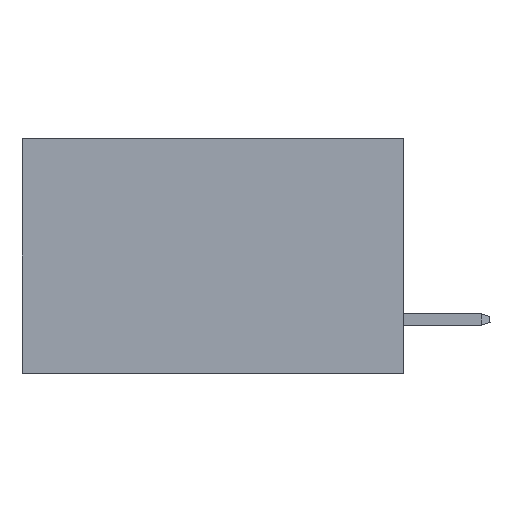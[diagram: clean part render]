
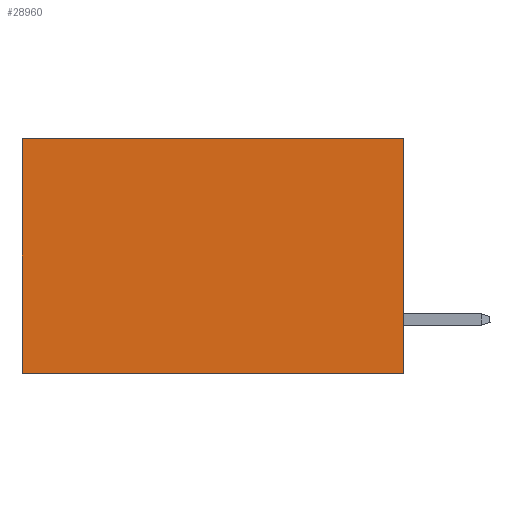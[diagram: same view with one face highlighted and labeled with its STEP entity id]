
A CAD part, left-side view. The second image highlights one B-rep face of the part: STEP entity #28960.
In plain terms, the highlighted planar face has unit normal (-1, 0, 0).
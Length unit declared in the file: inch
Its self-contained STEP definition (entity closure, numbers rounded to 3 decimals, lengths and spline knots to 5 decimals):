
#596 = DIRECTION ( 'NONE',  ( 0., 0., -1. ) ) ;
#1009 = FACE_OUTER_BOUND ( 'NONE', #10505, .T. ) ;
#2337 = VECTOR ( 'NONE', #19272, 39.37008 ) ;
#2617 = CARTESIAN_POINT ( 'NONE',  ( 0.2875, 0., -0.37 ) ) ;
#3300 = DIRECTION ( 'NONE',  ( 0., 1., 0. ) ) ;
#3303 = LINE ( 'NONE', #34037, #25437 ) ;
#3476 = LINE ( 'NONE', #6369, #29695 ) ;
#3677 = LINE ( 'NONE', #25749, #12272 ) ;
#5436 = ORIENTED_EDGE ( 'NONE', *, *, #15518, .F. ) ;
#6369 = CARTESIAN_POINT ( 'NONE',  ( 0.2875, 0., 0. ) ) ;
#6729 = DIRECTION ( 'NONE',  ( 0., 0., -1. ) ) ;
#9736 = VERTEX_POINT ( 'NONE', #25102 ) ;
#10505 = EDGE_LOOP ( 'NONE', ( #20571, #15126, #5436, #32160 ) ) ;
#12048 = DIRECTION ( 'NONE',  ( 0., 0., -1. ) ) ;
#12272 = VECTOR ( 'NONE', #6729, 39.37008 ) ;
#14213 = EDGE_CURVE ( 'NONE', #34789, #9736, #3303, .T. ) ;
#14393 = CARTESIAN_POINT ( 'NONE',  ( 0.2875, 0., -0.37 ) ) ;
#14777 = DIRECTION ( 'NONE',  ( 1., 0., 0. ) ) ;
#15126 = ORIENTED_EDGE ( 'NONE', *, *, #21246, .F. ) ;
#15299 = CARTESIAN_POINT ( 'NONE',  ( 0.2875, 0., 0. ) ) ;
#15518 = EDGE_CURVE ( 'NONE', #28375, #27790, #3677, .T. ) ;
#16241 = AXIS2_PLACEMENT_3D ( 'NONE', #15299, #14777, #12048 ) ;
#19272 = DIRECTION ( 'NONE',  ( 0., 1., 0. ) ) ;
#20571 = ORIENTED_EDGE ( 'NONE', *, *, #14213, .T. ) ;
#21246 = EDGE_CURVE ( 'NONE', #27790, #9736, #27397, .T. ) ;
#24232 = CARTESIAN_POINT ( 'NONE',  ( 0.2875, 0., 0. ) ) ;
#25102 = CARTESIAN_POINT ( 'NONE',  ( 0.2875, 0.6, -0.37 ) ) ;
#25437 = VECTOR ( 'NONE', #596, 39.37008 ) ;
#25749 = CARTESIAN_POINT ( 'NONE',  ( 0.2875, 0., 0. ) ) ;
#27397 = LINE ( 'NONE', #2617, #2337 ) ;
#27587 = CARTESIAN_POINT ( 'NONE',  ( 0.2875, 0.6, 0. ) ) ;
#27790 = VERTEX_POINT ( 'NONE', #14393 ) ;
#28375 = VERTEX_POINT ( 'NONE', #24232 ) ;
#28960 = ADVANCED_FACE ( 'NONE', ( #1009 ), #33913, .F. ) ;
#29695 = VECTOR ( 'NONE', #3300, 39.37008 ) ;
#32160 = ORIENTED_EDGE ( 'NONE', *, *, #32626, .T. ) ;
#32626 = EDGE_CURVE ( 'NONE', #28375, #34789, #3476, .T. ) ;
#33913 = PLANE ( 'NONE',  #16241 ) ;
#34037 = CARTESIAN_POINT ( 'NONE',  ( 0.2875, 0.6, 0. ) ) ;
#34789 = VERTEX_POINT ( 'NONE', #27587 ) ;
